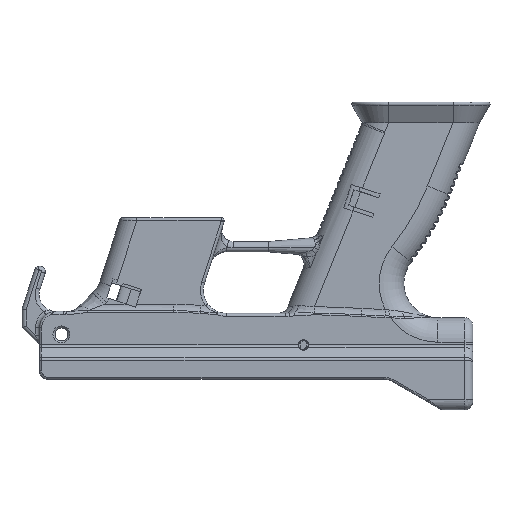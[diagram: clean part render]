
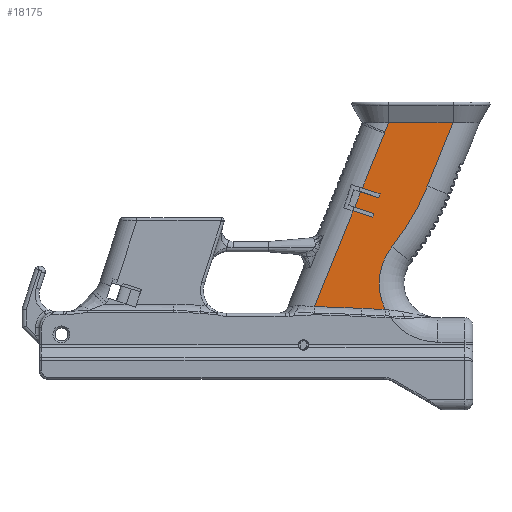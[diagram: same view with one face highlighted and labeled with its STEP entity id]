
A CAD part, front view. The second image highlights one B-rep face of the part: STEP entity #18175.
In plain terms, the highlighted planar face has unit normal (0, -1, 0).
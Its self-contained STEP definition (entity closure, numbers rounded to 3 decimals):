
#1740=FACE_OUTER_BOUND('',#2847,.T.);
#2847=EDGE_LOOP('',(#14018,#14019,#14020,#14021,#14022,#14023,#14024,#14025,
#14026,#14027,#14028,#14029,#14030,#14031,#14032,#14033,#14034));
#3870=CIRCLE('',#19895,696.304);
#3871=CIRCLE('',#19896,689.416);
#3872=CIRCLE('',#19897,28.63);
#3873=CIRCLE('',#19898,118.894);
#3874=CIRCLE('',#19899,17.);
#5504=LINE('',#32958,#6601);
#5519=LINE('',#33098,#6616);
#5520=LINE('',#33106,#6617);
#5562=LINE('',#34766,#6659);
#5563=LINE('',#34768,#6660);
#5564=LINE('',#34769,#6661);
#5565=LINE('',#34778,#6662);
#5566=LINE('',#34780,#6663);
#5567=LINE('',#34783,#6664);
#5568=LINE('',#34785,#6665);
#5569=LINE('',#34787,#6666);
#5570=LINE('',#34788,#6667);
#6601=VECTOR('',#23127,1000.);
#6616=VECTOR('',#23202,1000.);
#6617=VECTOR('',#23209,1000.);
#6659=VECTOR('',#23339,1000.);
#6660=VECTOR('',#23340,1000.);
#6661=VECTOR('',#23341,1000.);
#6662=VECTOR('',#23350,1000.);
#6663=VECTOR('',#23351,1000.);
#6664=VECTOR('',#23354,1000.);
#6665=VECTOR('',#23355,1000.);
#6666=VECTOR('',#23356,1000.);
#6667=VECTOR('',#23357,1000.);
#8272=VERTEX_POINT('',#32923);
#8274=VERTEX_POINT('',#32957);
#8300=VERTEX_POINT('',#33090);
#8301=VERTEX_POINT('',#33097);
#8304=VERTEX_POINT('',#33103);
#8305=VERTEX_POINT('',#33105);
#8387=VERTEX_POINT('',#34764);
#8388=VERTEX_POINT('',#34765);
#8389=VERTEX_POINT('',#34767);
#8390=VERTEX_POINT('',#34770);
#8391=VERTEX_POINT('',#34772);
#8392=VERTEX_POINT('',#34774);
#8393=VERTEX_POINT('',#34777);
#8394=VERTEX_POINT('',#34779);
#8395=VERTEX_POINT('',#34782);
#8396=VERTEX_POINT('',#34784);
#8397=VERTEX_POINT('',#34786);
#10403=EDGE_CURVE('',#8272,#8274,#5504,.T.);
#10445=EDGE_CURVE('',#8300,#8301,#5519,.T.);
#10449=EDGE_CURVE('',#8304,#8305,#5520,.T.);
#10578=EDGE_CURVE('',#8387,#8388,#5562,.T.);
#10579=EDGE_CURVE('',#8387,#8389,#5563,.T.);
#10580=EDGE_CURVE('',#8389,#8301,#5564,.T.);
#10581=EDGE_CURVE('',#8390,#8300,#3870,.T.);
#10582=EDGE_CURVE('',#8391,#8390,#3871,.T.);
#10583=EDGE_CURVE('',#8392,#8391,#3872,.T.);
#10584=EDGE_CURVE('',#8274,#8392,#3873,.T.);
#10585=EDGE_CURVE('',#8393,#8272,#5565,.T.);
#10586=EDGE_CURVE('',#8393,#8394,#5566,.T.);
#10587=EDGE_CURVE('',#8305,#8394,#3874,.T.);
#10588=EDGE_CURVE('',#8304,#8395,#5567,.T.);
#10589=EDGE_CURVE('',#8395,#8396,#5568,.T.);
#10590=EDGE_CURVE('',#8397,#8396,#5569,.T.);
#10591=EDGE_CURVE('',#8388,#8397,#5570,.T.);
#14018=ORIENTED_EDGE('',*,*,#10578,.F.);
#14019=ORIENTED_EDGE('',*,*,#10579,.T.);
#14020=ORIENTED_EDGE('',*,*,#10580,.T.);
#14021=ORIENTED_EDGE('',*,*,#10445,.F.);
#14022=ORIENTED_EDGE('',*,*,#10581,.F.);
#14023=ORIENTED_EDGE('',*,*,#10582,.F.);
#14024=ORIENTED_EDGE('',*,*,#10583,.F.);
#14025=ORIENTED_EDGE('',*,*,#10584,.F.);
#14026=ORIENTED_EDGE('',*,*,#10403,.F.);
#14027=ORIENTED_EDGE('',*,*,#10585,.F.);
#14028=ORIENTED_EDGE('',*,*,#10586,.T.);
#14029=ORIENTED_EDGE('',*,*,#10587,.F.);
#14030=ORIENTED_EDGE('',*,*,#10449,.F.);
#14031=ORIENTED_EDGE('',*,*,#10588,.T.);
#14032=ORIENTED_EDGE('',*,*,#10589,.T.);
#14033=ORIENTED_EDGE('',*,*,#10590,.F.);
#14034=ORIENTED_EDGE('',*,*,#10591,.F.);
#17565=PLANE('',#19894);
#18175=ADVANCED_FACE('',(#1740),#17565,.T.);
#19894=AXIS2_PLACEMENT_3D('',#34763,#23337,#23338);
#19895=AXIS2_PLACEMENT_3D('',#34771,#23342,#23343);
#19896=AXIS2_PLACEMENT_3D('',#34773,#23344,#23345);
#19897=AXIS2_PLACEMENT_3D('',#34775,#23346,#23347);
#19898=AXIS2_PLACEMENT_3D('',#34776,#23348,#23349);
#19899=AXIS2_PLACEMENT_3D('',#34781,#23352,#23353);
#23127=DIRECTION('',(-0.375,0.,-0.927));
#23202=DIRECTION('',(0.375,0.,0.927));
#23209=DIRECTION('',(0.375,0.,0.927));
#23337=DIRECTION('center_axis',(0.,-1.,0.));
#23338=DIRECTION('ref_axis',(0.,0.,-1.));
#23339=DIRECTION('',(-0.952,0.,0.305));
#23340=DIRECTION('',(-0.305,0.,-0.952));
#23341=DIRECTION('',(-0.952,0.,0.305));
#23342=DIRECTION('center_axis',(0.,-1.,0.));
#23343=DIRECTION('ref_axis',(-0.054,0.,-0.999));
#23344=DIRECTION('center_axis',(0.,1.,0.));
#23345=DIRECTION('ref_axis',(0.037,0.,0.999));
#23346=DIRECTION('center_axis',(0.,-1.,0.));
#23347=DIRECTION('ref_axis',(0.782,0.,-0.624));
#23348=DIRECTION('center_axis',(0.,1.,0.));
#23349=DIRECTION('ref_axis',(0.891,0.,-0.454));
#23350=DIRECTION('',(1.,0.,0.));
#23351=DIRECTION('',(-0.375,0.,-0.927));
#23352=DIRECTION('center_axis',(0.,-1.,0.));
#23353=DIRECTION('ref_axis',(0.992,0.,0.126));
#23354=DIRECTION('',(0.952,0.,-0.305));
#23355=DIRECTION('',(-0.305,0.,-0.952));
#23356=DIRECTION('',(0.952,0.,-0.305));
#23357=DIRECTION('',(0.375,0.,0.927));
#32923=CARTESIAN_POINT('',(121.365,-14.625,27.958));
#32957=CARTESIAN_POINT('',(108.893,-14.625,-2.912));
#32958=CARTESIAN_POINT('',(111.761,-14.625,4.188));
#33090=CARTESIAN_POINT('',(53.832,-14.625,-61.703));
#33097=CARTESIAN_POINT('',(72.662,-14.625,-15.097));
#33098=CARTESIAN_POINT('',(70.22,-14.625,-21.141));
#33103=CARTESIAN_POINT('',(77.169,-14.625,-3.94));
#33105=CARTESIAN_POINT('',(87.937,-14.625,22.71));
#33106=CARTESIAN_POINT('',(70.22,-14.625,-21.141));
#34763=CARTESIAN_POINT('Origin',(86.464,-14.625,-15.081));
#34764=CARTESIAN_POINT('',(82.782,-14.625,-16.238));
#34765=CARTESIAN_POINT('',(73.413,-14.625,-13.237));
#34766=CARTESIAN_POINT('',(2.985,-14.625,9.32));
#34767=CARTESIAN_POINT('',(82.172,-14.625,-18.143));
#34768=CARTESIAN_POINT('',(79.797,-14.625,-25.559));
#34769=CARTESIAN_POINT('',(2.375,-14.625,7.416));
#34770=CARTESIAN_POINT('',(76.954,-14.625,-62.561));
#34771=CARTESIAN_POINT('Origin',(39.557,-14.625,-757.86));
#34772=CARTESIAN_POINT('',(88.326,-14.625,-63.079));
#34773=CARTESIAN_POINT('Origin',(113.981,-14.625,625.86));
#34774=CARTESIAN_POINT('',(91.6,-14.625,-32.517));
#34775=CARTESIAN_POINT('Origin',(113.981,-14.625,-50.37));
#34776=CARTESIAN_POINT('Origin',(-1.344,-14.625,41.627));
#34777=CARTESIAN_POINT('',(90.04,-14.625,27.958));
#34778=CARTESIAN_POINT('',(69.665,-14.625,27.958));
#34779=CARTESIAN_POINT('',(88.199,-14.625,23.402));
#34780=CARTESIAN_POINT('',(106.929,-14.625,69.761));
#34781=CARTESIAN_POINT('Origin',(72.175,-14.625,29.078));
#34782=CARTESIAN_POINT('',(85.832,-14.625,-6.715));
#34783=CARTESIAN_POINT('',(88.836,-14.625,-7.677));
#34784=CARTESIAN_POINT('',(85.222,-14.625,-8.619));
#34785=CARTESIAN_POINT('',(79.797,-14.625,-25.559));
#34786=CARTESIAN_POINT('',(76.418,-14.625,-5.799));
#34787=CARTESIAN_POINT('',(88.226,-14.625,-9.581));
#34788=CARTESIAN_POINT('',(70.22,-14.625,-21.141));
